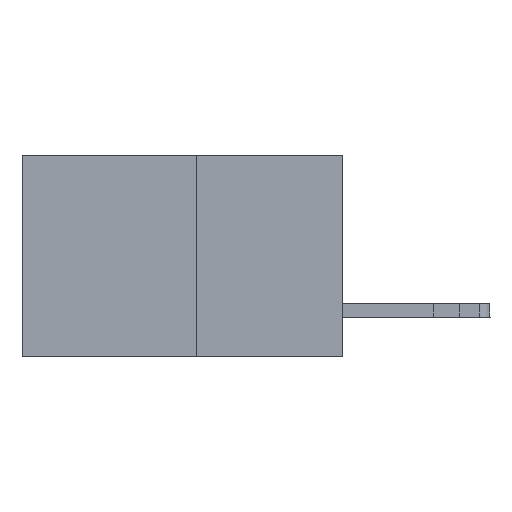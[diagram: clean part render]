
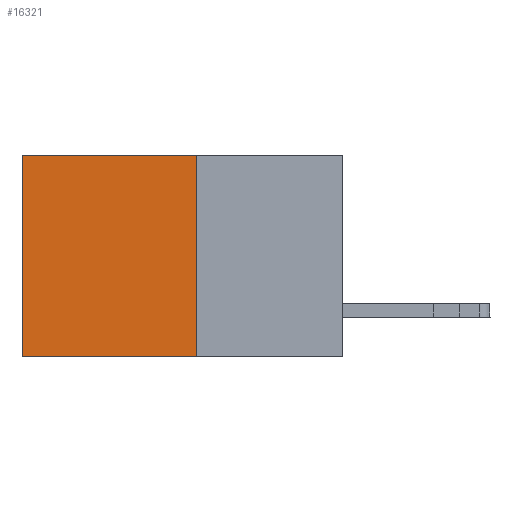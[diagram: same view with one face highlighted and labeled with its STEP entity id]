
A CAD part, left-side view. The second image highlights one B-rep face of the part: STEP entity #16321.
In plain terms, the highlighted planar face has unit normal (-1, 0, 0).
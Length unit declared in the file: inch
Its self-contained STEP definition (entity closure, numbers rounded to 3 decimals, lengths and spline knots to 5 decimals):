
#620 = ORIENTED_EDGE ( 'NONE', *, *, #3615, .F. ) ;
#717 = VERTEX_POINT ( 'NONE', #6351 ) ;
#746 = CARTESIAN_POINT ( 'NONE',  ( 0.277, 0.59, -0.37 ) ) ;
#1226 = LINE ( 'NONE', #7739, #9071 ) ;
#1246 = EDGE_CURVE ( 'NONE', #16584, #717, #2503, .T. ) ;
#1774 = EDGE_LOOP ( 'NONE', ( #11240, #620, #4288, #7904 ) ) ;
#2503 = LINE ( 'NONE', #5645, #4227 ) ;
#3615 = EDGE_CURVE ( 'NONE', #717, #18560, #15921, .T. ) ;
#4034 = CARTESIAN_POINT ( 'NONE',  ( 0.277, 0.27, -0.37 ) ) ;
#4227 = VECTOR ( 'NONE', #8911, 39.37008 ) ;
#4288 = ORIENTED_EDGE ( 'NONE', *, *, #1246, .F. ) ;
#5342 = DIRECTION ( 'NONE',  ( 0., 0., -1. ) ) ;
#5645 = CARTESIAN_POINT ( 'NONE',  ( 0.277, 0.27, -0.37 ) ) ;
#6203 = CARTESIAN_POINT ( 'NONE',  ( 0.277, 0.59, 0. ) ) ;
#6351 = CARTESIAN_POINT ( 'NONE',  ( 0.277, 0.27, -0.37 ) ) ;
#6489 = DIRECTION ( 'NONE',  ( 0., 1., 0. ) ) ;
#6967 = PLANE ( 'NONE',  #12374 ) ;
#7739 = CARTESIAN_POINT ( 'NONE',  ( 0.277, 0.27, 0. ) ) ;
#7904 = ORIENTED_EDGE ( 'NONE', *, *, #11553, .T. ) ;
#8703 = VECTOR ( 'NONE', #14244, 39.37008 ) ;
#8911 = DIRECTION ( 'NONE',  ( 0., 0., -1. ) ) ;
#9071 = VECTOR ( 'NONE', #14350, 39.37008 ) ;
#11240 = ORIENTED_EDGE ( 'NONE', *, *, #11308, .T. ) ;
#11308 = EDGE_CURVE ( 'NONE', #14805, #18560, #12193, .T. ) ;
#11553 = EDGE_CURVE ( 'NONE', #16584, #14805, #1226, .T. ) ;
#12067 = FACE_OUTER_BOUND ( 'NONE', #1774, .T. ) ;
#12193 = LINE ( 'NONE', #17159, #8703 ) ;
#12374 = AXIS2_PLACEMENT_3D ( 'NONE', #4034, #20156, #5342 ) ;
#14244 = DIRECTION ( 'NONE',  ( 0., 0., -1. ) ) ;
#14285 = CARTESIAN_POINT ( 'NONE',  ( 0.277, 0.27, 0. ) ) ;
#14350 = DIRECTION ( 'NONE',  ( 0., 1., 0. ) ) ;
#14805 = VERTEX_POINT ( 'NONE', #6203 ) ;
#15921 = LINE ( 'NONE', #17658, #17055 ) ;
#16321 = ADVANCED_FACE ( 'NONE', ( #12067 ), #6967, .F. ) ;
#16584 = VERTEX_POINT ( 'NONE', #14285 ) ;
#17055 = VECTOR ( 'NONE', #6489, 39.37008 ) ;
#17159 = CARTESIAN_POINT ( 'NONE',  ( 0.277, 0.59, -0.37 ) ) ;
#17658 = CARTESIAN_POINT ( 'NONE',  ( 0.277, 0.27, -0.37 ) ) ;
#18560 = VERTEX_POINT ( 'NONE', #746 ) ;
#20156 = DIRECTION ( 'NONE',  ( 1., 0., 0. ) ) ;
